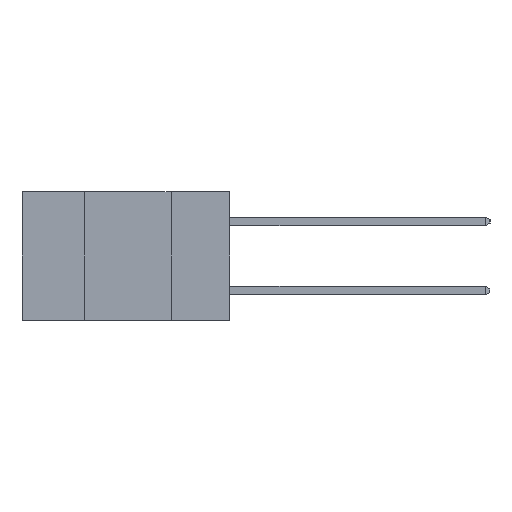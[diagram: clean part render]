
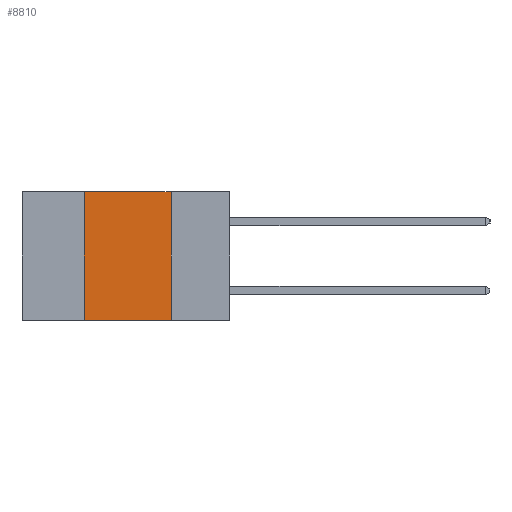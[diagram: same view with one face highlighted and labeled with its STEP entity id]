
A CAD part, left-side view. The second image highlights one B-rep face of the part: STEP entity #8810.
In plain terms, the highlighted planar face has unit normal (-1, 0, 0).
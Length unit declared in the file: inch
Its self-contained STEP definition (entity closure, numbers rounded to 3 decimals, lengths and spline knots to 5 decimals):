
#1013 = LINE ( 'NONE', #25277, #5594 ) ;
#1183 = VERTEX_POINT ( 'NONE', #4663 ) ;
#1427 = LINE ( 'NONE', #20708, #5393 ) ;
#1838 = VERTEX_POINT ( 'NONE', #15360 ) ;
#2128 = EDGE_CURVE ( 'NONE', #1183, #1838, #2144, .T. ) ;
#2144 = LINE ( 'NONE', #4948, #22375 ) ;
#3718 = EDGE_CURVE ( 'NONE', #11693, #8798, #11577, .T. ) ;
#4663 = CARTESIAN_POINT ( 'NONE',  ( 0., 0.17, 0. ) ) ;
#4948 = CARTESIAN_POINT ( 'NONE',  ( 0., 0.17, 0. ) ) ;
#5393 = VECTOR ( 'NONE', #12910, 39.37008 ) ;
#5594 = VECTOR ( 'NONE', #9669, 39.37008 ) ;
#6292 = DIRECTION ( 'NONE',  ( 0., 0., 1. ) ) ;
#8338 = FACE_OUTER_BOUND ( 'NONE', #10307, .T. ) ;
#8798 = VERTEX_POINT ( 'NONE', #16360 ) ;
#8810 = ADVANCED_FACE ( 'NONE', ( #8338 ), #22270, .F. ) ;
#8824 = DIRECTION ( 'NONE',  ( 0., 0., -1. ) ) ;
#9199 = EDGE_CURVE ( 'NONE', #8798, #1183, #1013, .T. ) ;
#9669 = DIRECTION ( 'NONE',  ( 0., -1., 0. ) ) ;
#10307 = EDGE_LOOP ( 'NONE', ( #13727, #18962, #24124, #24730 ) ) ;
#10545 = CARTESIAN_POINT ( 'NONE',  ( 0., 0.6, 0. ) ) ;
#10967 = VECTOR ( 'NONE', #6292, 39.37008 ) ;
#11577 = LINE ( 'NONE', #14145, #10967 ) ;
#11693 = VERTEX_POINT ( 'NONE', #22813 ) ;
#12497 = DIRECTION ( 'NONE',  ( 0., 0., -1. ) ) ;
#12910 = DIRECTION ( 'NONE',  ( 0., -1., 0. ) ) ;
#13727 = ORIENTED_EDGE ( 'NONE', *, *, #2128, .F. ) ;
#14145 = CARTESIAN_POINT ( 'NONE',  ( 0., 0.42, 0. ) ) ;
#15360 = CARTESIAN_POINT ( 'NONE',  ( 0., 0.17, -0.37 ) ) ;
#16360 = CARTESIAN_POINT ( 'NONE',  ( 0., 0.42, 0. ) ) ;
#16624 = AXIS2_PLACEMENT_3D ( 'NONE', #10545, #24215, #12497 ) ;
#18962 = ORIENTED_EDGE ( 'NONE', *, *, #9199, .F. ) ;
#20708 = CARTESIAN_POINT ( 'NONE',  ( 0., 0.6, -0.37 ) ) ;
#22270 = PLANE ( 'NONE',  #16624 ) ;
#22375 = VECTOR ( 'NONE', #8824, 39.37008 ) ;
#22813 = CARTESIAN_POINT ( 'NONE',  ( 0., 0.42, -0.37 ) ) ;
#24124 = ORIENTED_EDGE ( 'NONE', *, *, #3718, .F. ) ;
#24215 = DIRECTION ( 'NONE',  ( 1., 0., 0. ) ) ;
#24730 = ORIENTED_EDGE ( 'NONE', *, *, #25297, .T. ) ;
#25277 = CARTESIAN_POINT ( 'NONE',  ( 0., 0.6, 0. ) ) ;
#25297 = EDGE_CURVE ( 'NONE', #11693, #1838, #1427, .T. ) ;
